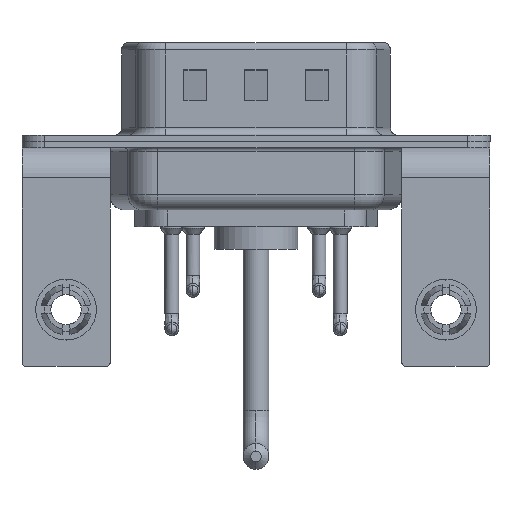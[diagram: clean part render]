
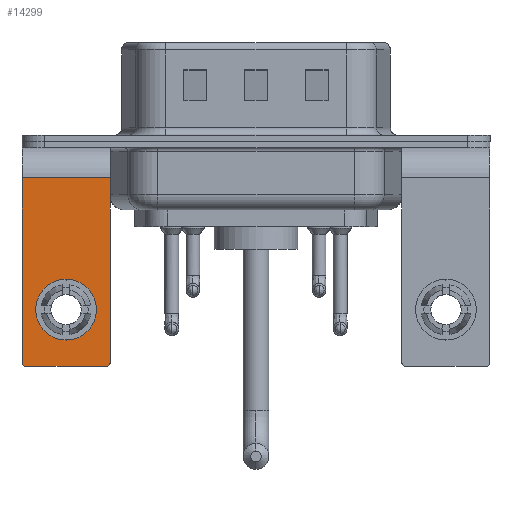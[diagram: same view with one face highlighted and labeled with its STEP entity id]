
A CAD part, front view. The second image highlights one B-rep face of the part: STEP entity #14299.
In plain terms, the highlighted planar face has unit normal (0, -1, 0).
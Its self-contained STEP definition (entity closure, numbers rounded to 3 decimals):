
#59 = ORIENTED_EDGE ( 'NONE', *, *, #3009, .T. ) ;
#123 = VERTEX_POINT ( 'NONE', #11794 ) ;
#816 = VECTOR ( 'NONE', #16499, 1000. ) ;
#1047 = VECTOR ( 'NONE', #20402, 1000. ) ;
#1401 = DIRECTION ( 'NONE',  ( 0., 1., 0. ) ) ;
#1738 = CARTESIAN_POINT ( 'NONE',  ( 2.9, -6.25, -14.8 ) ) ;
#1755 = AXIS2_PLACEMENT_3D ( 'NONE', #11595, #3236, #14881 ) ;
#1949 = ORIENTED_EDGE ( 'NONE', *, *, #3314, .T. ) ;
#2267 = EDGE_CURVE ( 'NONE', #20479, #17361, #3264, .T. ) ;
#2639 = VECTOR ( 'NONE', #14719, 1000. ) ;
#2693 = CIRCLE ( 'NONE', #10778, 0.25 ) ;
#2713 = CARTESIAN_POINT ( 'NONE',  ( 2.9, -6.25, -14.55 ) ) ;
#3009 = EDGE_CURVE ( 'NONE', #123, #13569, #2693, .T. ) ;
#3027 = CARTESIAN_POINT ( 'NONE',  ( 0., -6.25, -9.07 ) ) ;
#3236 = DIRECTION ( 'NONE',  ( 0., 1., 0. ) ) ;
#3264 = LINE ( 'NONE', #9965, #12455 ) ;
#3266 = CARTESIAN_POINT ( 'NONE',  ( 2.65, -6.25, -14.55 ) ) ;
#3314 = EDGE_CURVE ( 'NONE', #3645, #19451, #6232, .T. ) ;
#3645 = VERTEX_POINT ( 'NONE', #3027 ) ;
#4179 = CARTESIAN_POINT ( 'NONE',  ( -2.65, -6.25, -14.8 ) ) ;
#4184 = CARTESIAN_POINT ( 'NONE',  ( 0., -6.25, -11.07 ) ) ;
#5250 = ORIENTED_EDGE ( 'NONE', *, *, #2267, .F. ) ;
#5256 = VERTEX_POINT ( 'NONE', #8540 ) ;
#5868 = AXIS2_PLACEMENT_3D ( 'NONE', #13051, #1401, #21506 ) ;
#6232 = CIRCLE ( 'NONE', #11856, 2. ) ;
#6673 = EDGE_CURVE ( 'NONE', #20479, #5256, #9914, .T. ) ;
#7030 = EDGE_CURVE ( 'NONE', #5256, #123, #8222, .T. ) ;
#7630 = CARTESIAN_POINT ( 'NONE',  ( 2.9, -6.25, -2.4 ) ) ;
#7803 = DIRECTION ( 'NONE',  ( 0., 1., 0. ) ) ;
#8222 = LINE ( 'NONE', #17990, #2639 ) ;
#8292 = CARTESIAN_POINT ( 'NONE',  ( 0., -6.25, -13.07 ) ) ;
#8540 = CARTESIAN_POINT ( 'NONE',  ( -2.9, -6.25, -2.4 ) ) ;
#8619 = DIRECTION ( 'NONE',  ( 0., 0., -1. ) ) ;
#8723 = EDGE_LOOP ( 'NONE', ( #12691, #59, #11005, #16827, #5250, #16583 ) ) ;
#9219 = VERTEX_POINT ( 'NONE', #14896 ) ;
#9463 = CIRCLE ( 'NONE', #1755, 2. ) ;
#9914 = LINE ( 'NONE', #16382, #816 ) ;
#9965 = CARTESIAN_POINT ( 'NONE',  ( 2.9, -6.25, -2.4 ) ) ;
#10186 = FACE_OUTER_BOUND ( 'NONE', #8723, .T. ) ;
#10187 = DIRECTION ( 'NONE',  ( 0., 0., 1. ) ) ;
#10312 = DIRECTION ( 'NONE',  ( 0., -1., 0. ) ) ;
#10778 = AXIS2_PLACEMENT_3D ( 'NONE', #17995, #10312, #18325 ) ;
#11005 = ORIENTED_EDGE ( 'NONE', *, *, #20266, .F. ) ;
#11595 = CARTESIAN_POINT ( 'NONE',  ( 0., -6.25, -11.07 ) ) ;
#11794 = CARTESIAN_POINT ( 'NONE',  ( -2.9, -6.25, -14.55 ) ) ;
#11856 = AXIS2_PLACEMENT_3D ( 'NONE', #4184, #7803, #14625 ) ;
#12145 = LINE ( 'NONE', #1738, #1047 ) ;
#12455 = VECTOR ( 'NONE', #8619, 1000. ) ;
#12589 = CIRCLE ( 'NONE', #14352, 0.25 ) ;
#12691 = ORIENTED_EDGE ( 'NONE', *, *, #7030, .T. ) ;
#13051 = CARTESIAN_POINT ( 'NONE',  ( 2.9, -6.25, -2.4 ) ) ;
#13569 = VERTEX_POINT ( 'NONE', #4179 ) ;
#14299 = ADVANCED_FACE ( 'NONE', ( #18508, #10186 ), #21396, .F. ) ;
#14352 = AXIS2_PLACEMENT_3D ( 'NONE', #3266, #18509, #10187 ) ;
#14625 = DIRECTION ( 'NONE',  ( 0., 0., 1. ) ) ;
#14719 = DIRECTION ( 'NONE',  ( 0., 0., -1. ) ) ;
#14881 = DIRECTION ( 'NONE',  ( 0., 0., 1. ) ) ;
#14896 = CARTESIAN_POINT ( 'NONE',  ( 2.65, -6.25, -14.8 ) ) ;
#16382 = CARTESIAN_POINT ( 'NONE',  ( 2.9, -6.25, -2.4 ) ) ;
#16499 = DIRECTION ( 'NONE',  ( -1., 0., 0. ) ) ;
#16583 = ORIENTED_EDGE ( 'NONE', *, *, #6673, .T. ) ;
#16662 = EDGE_CURVE ( 'NONE', #19451, #3645, #9463, .T. ) ;
#16827 = ORIENTED_EDGE ( 'NONE', *, *, #17607, .T. ) ;
#17361 = VERTEX_POINT ( 'NONE', #2713 ) ;
#17399 = ORIENTED_EDGE ( 'NONE', *, *, #16662, .T. ) ;
#17607 = EDGE_CURVE ( 'NONE', #9219, #17361, #12589, .T. ) ;
#17990 = CARTESIAN_POINT ( 'NONE',  ( -2.9, -6.25, -2.4 ) ) ;
#17995 = CARTESIAN_POINT ( 'NONE',  ( -2.65, -6.25, -14.55 ) ) ;
#18325 = DIRECTION ( 'NONE',  ( 0., 0., 1. ) ) ;
#18508 = FACE_BOUND ( 'NONE', #18527, .T. ) ;
#18509 = DIRECTION ( 'NONE',  ( 0., -1., 0. ) ) ;
#18527 = EDGE_LOOP ( 'NONE', ( #17399, #1949 ) ) ;
#19451 = VERTEX_POINT ( 'NONE', #8292 ) ;
#20266 = EDGE_CURVE ( 'NONE', #9219, #13569, #12145, .T. ) ;
#20402 = DIRECTION ( 'NONE',  ( -1., 0., 0. ) ) ;
#20479 = VERTEX_POINT ( 'NONE', #7630 ) ;
#21396 = PLANE ( 'NONE',  #5868 ) ;
#21506 = DIRECTION ( 'NONE',  ( 0., 0., 1. ) ) ;
